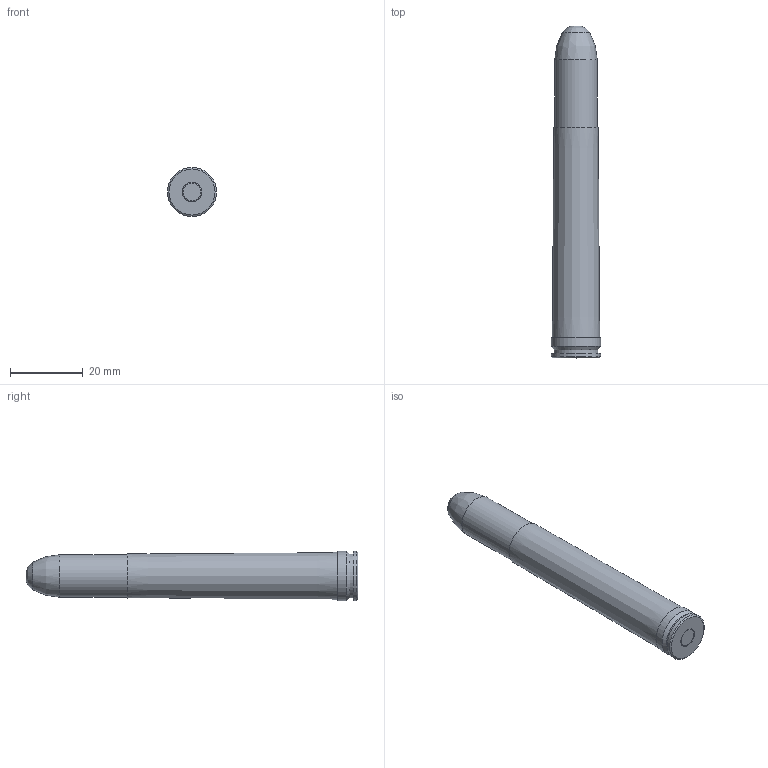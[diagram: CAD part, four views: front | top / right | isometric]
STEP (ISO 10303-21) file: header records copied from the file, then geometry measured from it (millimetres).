
FILE_DESCRIPTION((''),'2;1');
FILE_NAME('458 Lott.stp','2012-12-07T12:56:59',('agarrett'),(''),'Autodesk Inventor 2012','Autodesk Inventor 2012','');
FILE_SCHEMA(('AUTOMOTIVE_DESIGN { 1 0 10303 214 1 1 1 1 }'));
Length unit declared in the file: inch
Products named in the file (4): iLogic Cartridge; BeltedStraight; iLogic RN Bullet; PRIMER
Assembly tree (3 placements, depth 2):
  iLogic Cartridge
    BeltedStraight
    iLogic RN Bullet
    PRIMER
Bounding box: 13.51 x 91.44 x 13.51 mm (x, y, z)
Volume: 4907.4 mm3; surface area: 6804 mm2
Topology: 3 solids, 3 shells, 29 faces, 45 edges, 27 vertices
Faces by surface type: plane 11, cylinder 8, cone 4, torus 4, bspline 2
Full cylindrical faces by diameter (mm): 1.778 x1, 5.08 x1, 5.334 x2, 11.661 x1, 12.07 x1, 13.51 x2
Entity records: 760 total; most frequent: CARTESIAN_POINT 142, DIRECTION 122, AXIS2_PLACEMENT_3D 61, ORIENTED_EDGE 54, EDGE_LOOP 54, FACE_OUTER_BOUND 29, ADVANCED_FACE 29, VERTEX_POINT 27
